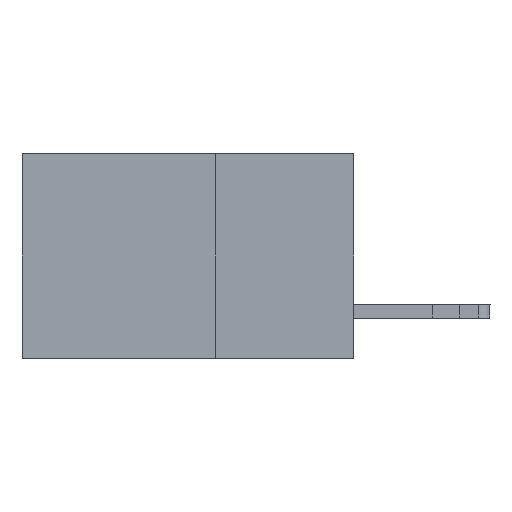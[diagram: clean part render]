
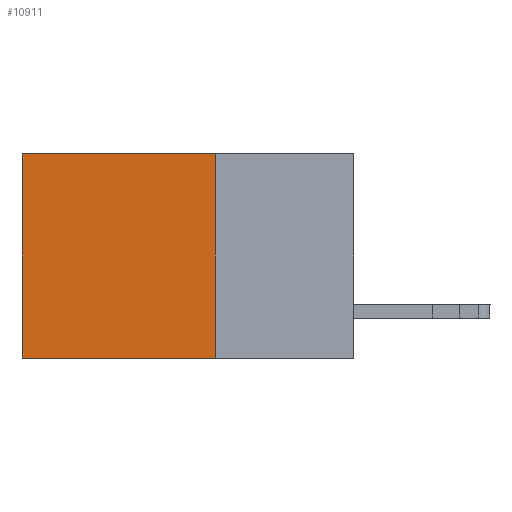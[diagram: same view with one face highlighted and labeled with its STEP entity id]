
A CAD part, left-side view. The second image highlights one B-rep face of the part: STEP entity #10911.
In plain terms, the highlighted planar face has unit normal (-1, 0, 0).
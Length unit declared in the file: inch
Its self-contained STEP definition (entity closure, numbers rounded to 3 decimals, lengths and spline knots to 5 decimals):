
#285 = EDGE_CURVE ( 'NONE', #16783, #9084, #3802, .T. ) ;
#464 = VERTEX_POINT ( 'NONE', #8165 ) ;
#503 = CARTESIAN_POINT ( 'NONE',  ( 0.2875, 0.25, -0.37 ) ) ;
#523 = LINE ( 'NONE', #2608, #8710 ) ;
#717 = DIRECTION ( 'NONE',  ( 0., 1., 0. ) ) ;
#777 = ORIENTED_EDGE ( 'NONE', *, *, #3937, .T. ) ;
#2197 = DIRECTION ( 'NONE',  ( 0., 0., -1. ) ) ;
#2377 = PLANE ( 'NONE',  #15019 ) ;
#2608 = CARTESIAN_POINT ( 'NONE',  ( 0.2875, 0.25, -0.37 ) ) ;
#3336 = ORIENTED_EDGE ( 'NONE', *, *, #14930, .T. ) ;
#3511 = EDGE_CURVE ( 'NONE', #9084, #464, #523, .T. ) ;
#3802 = LINE ( 'NONE', #8689, #6573 ) ;
#3937 = EDGE_CURVE ( 'NONE', #7671, #464, #4491, .T. ) ;
#4491 = LINE ( 'NONE', #13414, #8690 ) ;
#4756 = CARTESIAN_POINT ( 'NONE',  ( 0.2875, 0.25, 0. ) ) ;
#5013 = CARTESIAN_POINT ( 'NONE',  ( 0.2875, 0.25, 0. ) ) ;
#5713 = EDGE_LOOP ( 'NONE', ( #777, #7910, #16108, #3336 ) ) ;
#5956 = CARTESIAN_POINT ( 'NONE',  ( 0.2875, 0.25, 0. ) ) ;
#6573 = VECTOR ( 'NONE', #14047, 39.37008 ) ;
#7671 = VERTEX_POINT ( 'NONE', #9563 ) ;
#7910 = ORIENTED_EDGE ( 'NONE', *, *, #3511, .F. ) ;
#8032 = DIRECTION ( 'NONE',  ( 0., 0., -1. ) ) ;
#8165 = CARTESIAN_POINT ( 'NONE',  ( 0.2875, 0.6, -0.37 ) ) ;
#8689 = CARTESIAN_POINT ( 'NONE',  ( 0.2875, 0.25, 0. ) ) ;
#8690 = VECTOR ( 'NONE', #8032, 39.37008 ) ;
#8710 = VECTOR ( 'NONE', #9100, 39.37008 ) ;
#9084 = VERTEX_POINT ( 'NONE', #503 ) ;
#9100 = DIRECTION ( 'NONE',  ( 0., 1., 0. ) ) ;
#9563 = CARTESIAN_POINT ( 'NONE',  ( 0.2875, 0.6, 0. ) ) ;
#10911 = ADVANCED_FACE ( 'NONE', ( #12070 ), #2377, .F. ) ;
#12070 = FACE_OUTER_BOUND ( 'NONE', #5713, .T. ) ;
#12835 = VECTOR ( 'NONE', #717, 39.37008 ) ;
#13414 = CARTESIAN_POINT ( 'NONE',  ( 0.2875, 0.6, 0. ) ) ;
#14047 = DIRECTION ( 'NONE',  ( 0., 0., -1. ) ) ;
#14132 = DIRECTION ( 'NONE',  ( 1., 0., 0. ) ) ;
#14475 = LINE ( 'NONE', #4756, #12835 ) ;
#14930 = EDGE_CURVE ( 'NONE', #16783, #7671, #14475, .T. ) ;
#15019 = AXIS2_PLACEMENT_3D ( 'NONE', #5013, #14132, #2197 ) ;
#16108 = ORIENTED_EDGE ( 'NONE', *, *, #285, .F. ) ;
#16783 = VERTEX_POINT ( 'NONE', #5956 ) ;
